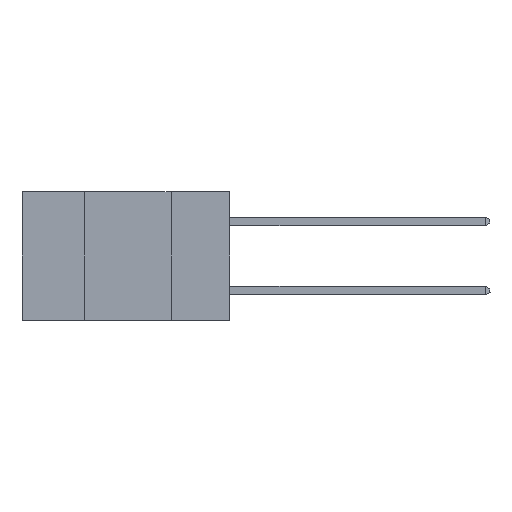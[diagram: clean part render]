
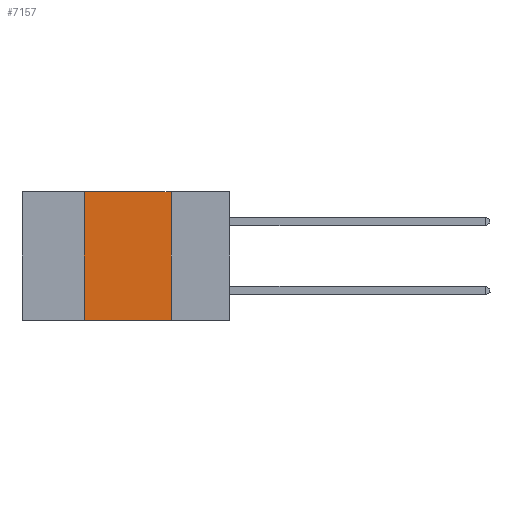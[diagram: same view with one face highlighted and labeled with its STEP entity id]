
A CAD part, left-side view. The second image highlights one B-rep face of the part: STEP entity #7157.
In plain terms, the highlighted planar face has unit normal (-1, 0, 0).
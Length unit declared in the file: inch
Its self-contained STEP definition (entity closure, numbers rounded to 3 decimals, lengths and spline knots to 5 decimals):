
#52 = EDGE_CURVE ( 'NONE', #9446, #1745, #14277, .T. ) ;
#109 = EDGE_CURVE ( 'NONE', #11942, #6800, #7481, .T. ) ;
#141 = CARTESIAN_POINT ( 'NONE',  ( 0., 0.6, 0. ) ) ;
#492 = VECTOR ( 'NONE', #5642, 39.37008 ) ;
#508 = DIRECTION ( 'NONE',  ( 1., 0., 0. ) ) ;
#666 = DIRECTION ( 'NONE',  ( 0., 0., -1. ) ) ;
#962 = AXIS2_PLACEMENT_3D ( 'NONE', #12830, #508, #666 ) ;
#1004 = CARTESIAN_POINT ( 'NONE',  ( 0., 0.42, 0. ) ) ;
#1561 = VECTOR ( 'NONE', #13756, 39.37008 ) ;
#1745 = VERTEX_POINT ( 'NONE', #10338 ) ;
#1829 = EDGE_LOOP ( 'NONE', ( #9384, #11130, #12192, #13405 ) ) ;
#2377 = VECTOR ( 'NONE', #13467, 39.37008 ) ;
#3193 = EDGE_CURVE ( 'NONE', #11942, #9446, #9861, .T. ) ;
#3341 = CARTESIAN_POINT ( 'NONE',  ( 0., 0.42, -0.37 ) ) ;
#5076 = LINE ( 'NONE', #10788, #6459 ) ;
#5399 = DIRECTION ( 'NONE',  ( 0., 0., -1. ) ) ;
#5642 = DIRECTION ( 'NONE',  ( 0., -1., 0. ) ) ;
#6459 = VECTOR ( 'NONE', #5399, 39.37008 ) ;
#6800 = VERTEX_POINT ( 'NONE', #13040 ) ;
#6978 = CARTESIAN_POINT ( 'NONE',  ( 0., 0.6, -0.37 ) ) ;
#7157 = ADVANCED_FACE ( 'NONE', ( #8855 ), #11837, .F. ) ;
#7244 = EDGE_CURVE ( 'NONE', #1745, #6800, #5076, .T. ) ;
#7481 = LINE ( 'NONE', #6978, #1561 ) ;
#7873 = CARTESIAN_POINT ( 'NONE',  ( 0., 0.42, 0. ) ) ;
#8855 = FACE_OUTER_BOUND ( 'NONE', #1829, .T. ) ;
#9384 = ORIENTED_EDGE ( 'NONE', *, *, #7244, .F. ) ;
#9446 = VERTEX_POINT ( 'NONE', #1004 ) ;
#9861 = LINE ( 'NONE', #7873, #2377 ) ;
#10338 = CARTESIAN_POINT ( 'NONE',  ( 0., 0.17, 0. ) ) ;
#10788 = CARTESIAN_POINT ( 'NONE',  ( 0., 0.17, 0. ) ) ;
#11130 = ORIENTED_EDGE ( 'NONE', *, *, #52, .F. ) ;
#11837 = PLANE ( 'NONE',  #962 ) ;
#11942 = VERTEX_POINT ( 'NONE', #3341 ) ;
#12192 = ORIENTED_EDGE ( 'NONE', *, *, #3193, .F. ) ;
#12830 = CARTESIAN_POINT ( 'NONE',  ( 0., 0.6, 0. ) ) ;
#13040 = CARTESIAN_POINT ( 'NONE',  ( 0., 0.17, -0.37 ) ) ;
#13405 = ORIENTED_EDGE ( 'NONE', *, *, #109, .T. ) ;
#13467 = DIRECTION ( 'NONE',  ( 0., 0., 1. ) ) ;
#13756 = DIRECTION ( 'NONE',  ( 0., -1., 0. ) ) ;
#14277 = LINE ( 'NONE', #141, #492 ) ;
